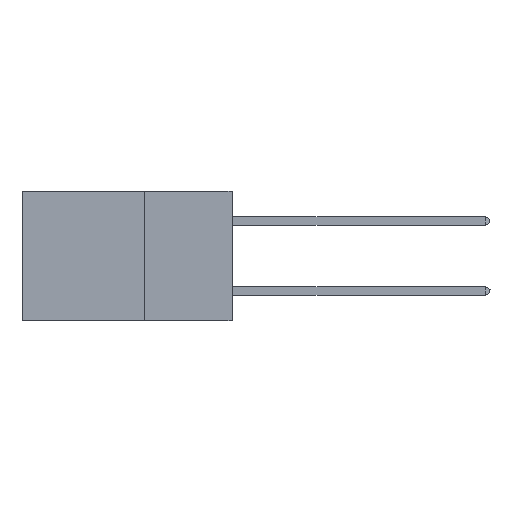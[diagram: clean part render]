
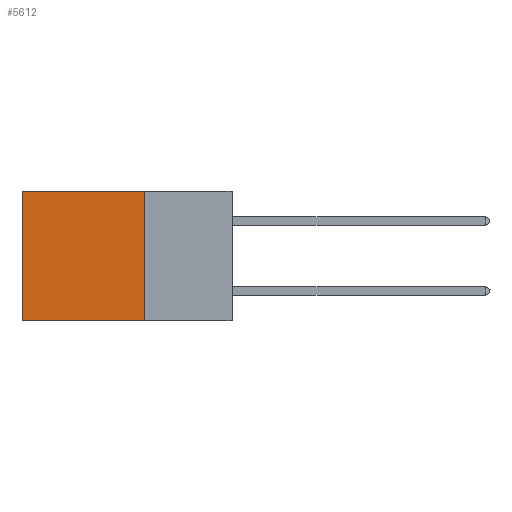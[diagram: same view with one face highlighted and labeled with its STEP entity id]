
A CAD part, left-side view. The second image highlights one B-rep face of the part: STEP entity #5612.
In plain terms, the highlighted planar face has unit normal (-1, 0, 0).
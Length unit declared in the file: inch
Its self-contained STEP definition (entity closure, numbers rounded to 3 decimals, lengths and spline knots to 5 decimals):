
#62 = LINE ( 'NONE', #9868, #17630 ) ;
#270 = DIRECTION ( 'NONE',  ( 0., 0., -1. ) ) ;
#657 = DIRECTION ( 'NONE',  ( 1., 0., 0. ) ) ;
#1161 = CARTESIAN_POINT ( 'NONE',  ( 0.2875, 0.6, -0.37 ) ) ;
#2015 = DIRECTION ( 'NONE',  ( 0., 0., -1. ) ) ;
#2181 = LINE ( 'NONE', #17797, #15712 ) ;
#2386 = VERTEX_POINT ( 'NONE', #1161 ) ;
#2801 = VERTEX_POINT ( 'NONE', #13206 ) ;
#3309 = ORIENTED_EDGE ( 'NONE', *, *, #7618, .T. ) ;
#3702 = FACE_OUTER_BOUND ( 'NONE', #15058, .T. ) ;
#3859 = VERTEX_POINT ( 'NONE', #8610 ) ;
#4144 = VERTEX_POINT ( 'NONE', #8015 ) ;
#4162 = DIRECTION ( 'NONE',  ( 0., 1., 0. ) ) ;
#4565 = EDGE_CURVE ( 'NONE', #4144, #2386, #7891, .T. ) ;
#5260 = AXIS2_PLACEMENT_3D ( 'NONE', #16151, #657, #2015 ) ;
#5612 = ADVANCED_FACE ( 'NONE', ( #3702 ), #14446, .F. ) ;
#7618 = EDGE_CURVE ( 'NONE', #3859, #2801, #62, .T. ) ;
#7891 = LINE ( 'NONE', #9458, #15425 ) ;
#7956 = LINE ( 'NONE', #14864, #18573 ) ;
#8015 = CARTESIAN_POINT ( 'NONE',  ( 0.2875, 0.25, -0.37 ) ) ;
#8610 = CARTESIAN_POINT ( 'NONE',  ( 0.2875, 0.25, 0. ) ) ;
#9458 = CARTESIAN_POINT ( 'NONE',  ( 0.2875, 0.25, -0.37 ) ) ;
#9868 = CARTESIAN_POINT ( 'NONE',  ( 0.2875, 0.25, 0. ) ) ;
#10535 = ORIENTED_EDGE ( 'NONE', *, *, #18861, .T. ) ;
#13206 = CARTESIAN_POINT ( 'NONE',  ( 0.2875, 0.6, 0. ) ) ;
#14370 = ORIENTED_EDGE ( 'NONE', *, *, #16474, .F. ) ;
#14446 = PLANE ( 'NONE',  #5260 ) ;
#14864 = CARTESIAN_POINT ( 'NONE',  ( 0.2875, 0.6, 0. ) ) ;
#15058 = EDGE_LOOP ( 'NONE', ( #10535, #16603, #14370, #3309 ) ) ;
#15425 = VECTOR ( 'NONE', #4162, 39.37008 ) ;
#15712 = VECTOR ( 'NONE', #270, 39.37008 ) ;
#16151 = CARTESIAN_POINT ( 'NONE',  ( 0.2875, 0.25, 0. ) ) ;
#16474 = EDGE_CURVE ( 'NONE', #3859, #4144, #2181, .T. ) ;
#16603 = ORIENTED_EDGE ( 'NONE', *, *, #4565, .F. ) ;
#17630 = VECTOR ( 'NONE', #22037, 39.37008 ) ;
#17797 = CARTESIAN_POINT ( 'NONE',  ( 0.2875, 0.25, 0. ) ) ;
#18573 = VECTOR ( 'NONE', #22137, 39.37008 ) ;
#18861 = EDGE_CURVE ( 'NONE', #2801, #2386, #7956, .T. ) ;
#22037 = DIRECTION ( 'NONE',  ( 0., 1., 0. ) ) ;
#22137 = DIRECTION ( 'NONE',  ( 0., 0., -1. ) ) ;
